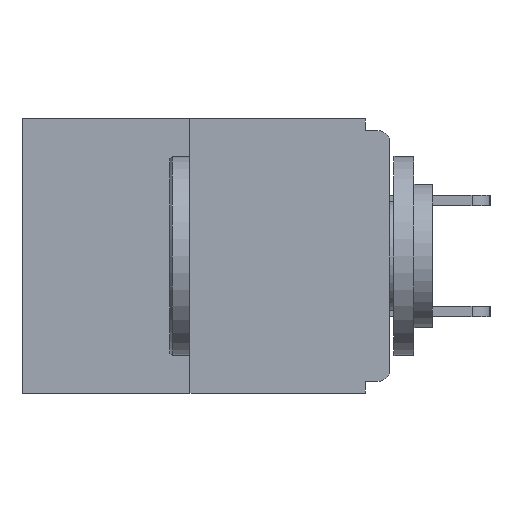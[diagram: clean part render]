
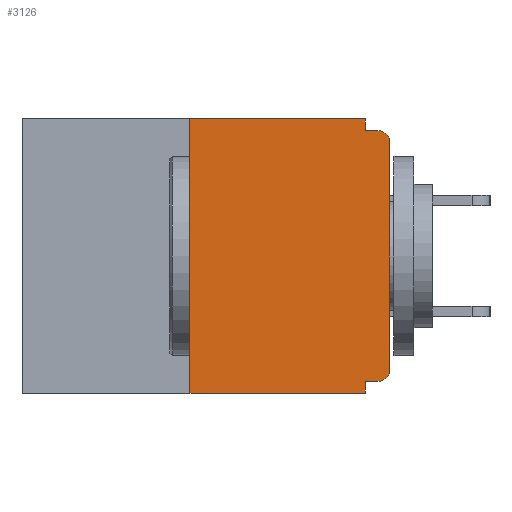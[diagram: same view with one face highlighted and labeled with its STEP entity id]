
A CAD part, left-side view. The second image highlights one B-rep face of the part: STEP entity #3126.
In plain terms, the highlighted planar face has unit normal (-1, 0, 0).
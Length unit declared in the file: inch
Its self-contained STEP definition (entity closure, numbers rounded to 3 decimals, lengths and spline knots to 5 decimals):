
#309 = CARTESIAN_POINT ( 'NONE',  ( 0., 0.46, 0. ) ) ;
#1153 = CARTESIAN_POINT ( 'NONE',  ( 0., 0., -0.328 ) ) ;
#1872 = ORIENTED_EDGE ( 'NONE', *, *, #6399, .F. ) ;
#1967 = CARTESIAN_POINT ( 'NONE',  ( 0., 0.25, 0. ) ) ;
#2112 = AXIS2_PLACEMENT_3D ( 'NONE', #8281, #13244, #17875 ) ;
#2227 = CARTESIAN_POINT ( 'NONE',  ( 0., 0.46, -0.343 ) ) ;
#2328 = CARTESIAN_POINT ( 'NONE',  ( 0., 0.031, -0.343 ) ) ;
#2413 = EDGE_CURVE ( 'NONE', #28420, #4766, #20660, .T. ) ;
#2557 = VECTOR ( 'NONE', #17127, 39.37008 ) ;
#2643 = DIRECTION ( 'NONE',  ( 0., 0., -1. ) ) ;
#2648 = DIRECTION ( 'NONE',  ( 0., 0., -1. ) ) ;
#3022 = VECTOR ( 'NONE', #8402, 39.37008 ) ;
#3126 = ADVANCED_FACE ( 'NONE', ( #28409 ), #5336, .F. ) ;
#3711 = CARTESIAN_POINT ( 'NONE',  ( 0., 0., -0.03 ) ) ;
#3836 = LINE ( 'NONE', #2328, #21201 ) ;
#4074 = CARTESIAN_POINT ( 'NONE',  ( 0., 0., -0.313 ) ) ;
#4766 = VERTEX_POINT ( 'NONE', #20362 ) ;
#5160 = CARTESIAN_POINT ( 'NONE',  ( 0., 0.25, 0. ) ) ;
#5336 = PLANE ( 'NONE',  #28747 ) ;
#6399 = EDGE_CURVE ( 'NONE', #23849, #4766, #3836, .T. ) ;
#6652 = VERTEX_POINT ( 'NONE', #27633 ) ;
#7670 = LINE ( 'NONE', #23047, #15386 ) ;
#8281 = CARTESIAN_POINT ( 'NONE',  ( 0., 0.015, -0.03 ) ) ;
#8402 = DIRECTION ( 'NONE',  ( 0., 1., 0. ) ) ;
#8756 = ORIENTED_EDGE ( 'NONE', *, *, #21136, .F. ) ;
#10344 = VERTEX_POINT ( 'NONE', #12448 ) ;
#10419 = EDGE_CURVE ( 'NONE', #11838, #6652, #18267, .T. ) ;
#11045 = ORIENTED_EDGE ( 'NONE', *, *, #16186, .T. ) ;
#11443 = ORIENTED_EDGE ( 'NONE', *, *, #29920, .T. ) ;
#11838 = VERTEX_POINT ( 'NONE', #1967 ) ;
#12303 = CARTESIAN_POINT ( 'NONE',  ( 0., 0., -0.015 ) ) ;
#12372 = LINE ( 'NONE', #25059, #24713 ) ;
#12448 = CARTESIAN_POINT ( 'NONE',  ( 0., 0.015, -0.328 ) ) ;
#13231 = VECTOR ( 'NONE', #29646, 39.37008 ) ;
#13244 = DIRECTION ( 'NONE',  ( -1., 0., 0. ) ) ;
#13248 = DIRECTION ( 'NONE',  ( 0., 0., -1. ) ) ;
#13411 = AXIS2_PLACEMENT_3D ( 'NONE', #21392, #26350, #28867 ) ;
#13455 = ORIENTED_EDGE ( 'NONE', *, *, #20078, .F. ) ;
#14954 = CARTESIAN_POINT ( 'NONE',  ( 0., 0.46, 0. ) ) ;
#15145 = VECTOR ( 'NONE', #17607, 39.37008 ) ;
#15194 = DIRECTION ( 'NONE',  ( 0., 0., 1. ) ) ;
#15250 = CARTESIAN_POINT ( 'NONE',  ( 0., 0.031, -0.015 ) ) ;
#15386 = VECTOR ( 'NONE', #13248, 39.37008 ) ;
#16186 = EDGE_CURVE ( 'NONE', #29905, #28037, #19470, .T. ) ;
#16628 = ORIENTED_EDGE ( 'NONE', *, *, #17261, .F. ) ;
#16695 = LINE ( 'NONE', #12303, #13231 ) ;
#17127 = DIRECTION ( 'NONE',  ( 0., -1., 0. ) ) ;
#17182 = VERTEX_POINT ( 'NONE', #4074 ) ;
#17261 = EDGE_CURVE ( 'NONE', #24565, #28037, #16695, .T. ) ;
#17607 = DIRECTION ( 'NONE',  ( 0., -1., 0. ) ) ;
#17875 = DIRECTION ( 'NONE',  ( 0., 0., -1. ) ) ;
#18267 = LINE ( 'NONE', #309, #15145 ) ;
#19088 = VECTOR ( 'NONE', #15194, 39.37008 ) ;
#19470 = CIRCLE ( 'NONE', #2112, 0.015 ) ;
#20078 = EDGE_CURVE ( 'NONE', #6652, #24565, #7670, .T. ) ;
#20362 = CARTESIAN_POINT ( 'NONE',  ( 0., 0.031, -0.343 ) ) ;
#20377 = ORIENTED_EDGE ( 'NONE', *, *, #20492, .T. ) ;
#20492 = EDGE_CURVE ( 'NONE', #17182, #29905, #12372, .T. ) ;
#20660 = LINE ( 'NONE', #2227, #2557 ) ;
#20694 = CIRCLE ( 'NONE', #13411, 0.015 ) ;
#21012 = LINE ( 'NONE', #5160, #19088 ) ;
#21136 = EDGE_CURVE ( 'NONE', #10344, #23849, #29664, .T. ) ;
#21201 = VECTOR ( 'NONE', #2643, 39.37008 ) ;
#21392 = CARTESIAN_POINT ( 'NONE',  ( 0., 0.015, -0.313 ) ) ;
#22046 = CARTESIAN_POINT ( 'NONE',  ( 0., 0.031, -0.328 ) ) ;
#22685 = DIRECTION ( 'NONE',  ( 1., 0., 0. ) ) ;
#23047 = CARTESIAN_POINT ( 'NONE',  ( 0., 0.031, 0. ) ) ;
#23849 = VERTEX_POINT ( 'NONE', #22046 ) ;
#24047 = CARTESIAN_POINT ( 'NONE',  ( 0., 0.015, -0.015 ) ) ;
#24565 = VERTEX_POINT ( 'NONE', #15250 ) ;
#24713 = VECTOR ( 'NONE', #27631, 39.37008 ) ;
#25059 = CARTESIAN_POINT ( 'NONE',  ( 0., 0., 0. ) ) ;
#25617 = CARTESIAN_POINT ( 'NONE',  ( 0., 0.25, -0.343 ) ) ;
#26135 = ORIENTED_EDGE ( 'NONE', *, *, #10419, .F. ) ;
#26350 = DIRECTION ( 'NONE',  ( -1., 0., 0. ) ) ;
#27142 = ORIENTED_EDGE ( 'NONE', *, *, #2413, .T. ) ;
#27600 = EDGE_LOOP ( 'NONE', ( #26135, #29576, #27142, #1872, #8756, #11443, #20377, #11045, #16628, #13455 ) ) ;
#27631 = DIRECTION ( 'NONE',  ( 0., 0., 1. ) ) ;
#27633 = CARTESIAN_POINT ( 'NONE',  ( 0., 0.031, 0. ) ) ;
#28037 = VERTEX_POINT ( 'NONE', #24047 ) ;
#28409 = FACE_OUTER_BOUND ( 'NONE', #27600, .T. ) ;
#28420 = VERTEX_POINT ( 'NONE', #25617 ) ;
#28747 = AXIS2_PLACEMENT_3D ( 'NONE', #14954, #22685, #2648 ) ;
#28867 = DIRECTION ( 'NONE',  ( 0., 0., -1. ) ) ;
#29576 = ORIENTED_EDGE ( 'NONE', *, *, #30805, .F. ) ;
#29646 = DIRECTION ( 'NONE',  ( 0., -1., 0. ) ) ;
#29664 = LINE ( 'NONE', #1153, #3022 ) ;
#29905 = VERTEX_POINT ( 'NONE', #3711 ) ;
#29920 = EDGE_CURVE ( 'NONE', #10344, #17182, #20694, .T. ) ;
#30805 = EDGE_CURVE ( 'NONE', #28420, #11838, #21012, .T. ) ;
